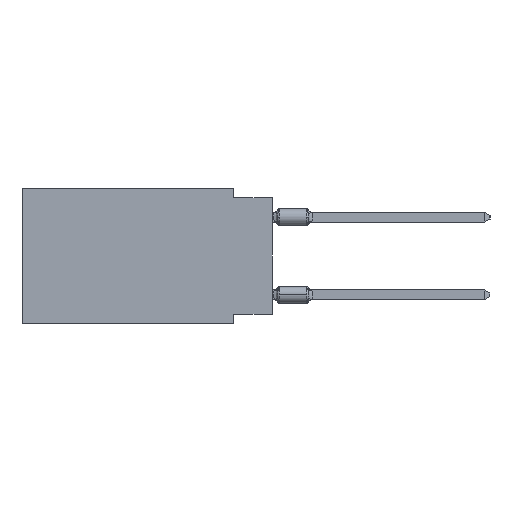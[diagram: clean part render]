
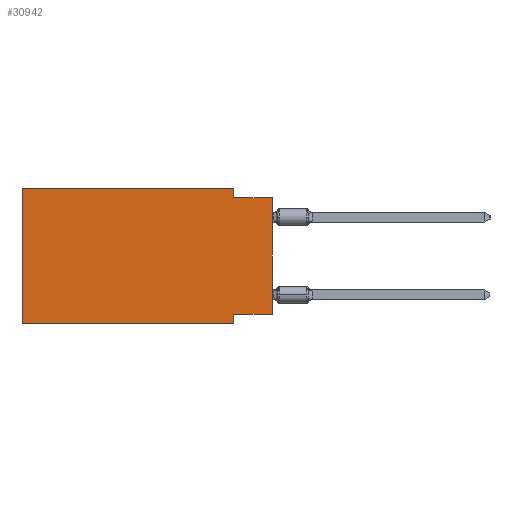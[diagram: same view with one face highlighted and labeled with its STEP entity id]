
A CAD part, left-side view. The second image highlights one B-rep face of the part: STEP entity #30942.
In plain terms, the highlighted planar face has unit normal (-1, 0, 0).
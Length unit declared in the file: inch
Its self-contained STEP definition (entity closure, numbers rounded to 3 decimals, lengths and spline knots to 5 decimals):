
#561 = AXIS2_PLACEMENT_3D ( 'NONE', #1893, #31019, #17840 ) ;
#577 = EDGE_CURVE ( 'NONE', #6546, #15256, #30887, .T. ) ;
#796 = EDGE_CURVE ( 'NONE', #6546, #3663, #32170, .T. ) ;
#1893 = CARTESIAN_POINT ( 'NONE',  ( 0., 0.645, 0. ) ) ;
#2189 = EDGE_LOOP ( 'NONE', ( #30803, #37781, #32144, #37199, #9727, #32442, #23612, #23985 ) ) ;
#2251 = CARTESIAN_POINT ( 'NONE',  ( 0., 0.645, -0.35 ) ) ;
#3054 = EDGE_CURVE ( 'NONE', #3663, #24401, #9322, .T. ) ;
#3663 = VERTEX_POINT ( 'NONE', #26850 ) ;
#4867 = FACE_OUTER_BOUND ( 'NONE', #2189, .T. ) ;
#5063 = DIRECTION ( 'NONE',  ( 0., 0., -1. ) ) ;
#6546 = VERTEX_POINT ( 'NONE', #2251 ) ;
#7403 = VECTOR ( 'NONE', #8085, 39.37008 ) ;
#8085 = DIRECTION ( 'NONE',  ( 0., 1., 0. ) ) ;
#9322 = LINE ( 'NONE', #28452, #16639 ) ;
#9586 = CARTESIAN_POINT ( 'NONE',  ( 0., 0.1, -0.025 ) ) ;
#9727 = ORIENTED_EDGE ( 'NONE', *, *, #796, .F. ) ;
#10822 = DIRECTION ( 'NONE',  ( 0., 0., 1. ) ) ;
#10855 = VECTOR ( 'NONE', #23421, 39.37008 ) ;
#11446 = CARTESIAN_POINT ( 'NONE',  ( 0., 0., 0. ) ) ;
#13526 = DIRECTION ( 'NONE',  ( 0., -1., 0. ) ) ;
#13620 = VERTEX_POINT ( 'NONE', #9586 ) ;
#13847 = CARTESIAN_POINT ( 'NONE',  ( 0., 0.645, 0. ) ) ;
#14323 = VECTOR ( 'NONE', #10822, 39.37008 ) ;
#14880 = VERTEX_POINT ( 'NONE', #41095 ) ;
#15256 = VERTEX_POINT ( 'NONE', #16311 ) ;
#15702 = DIRECTION ( 'NONE',  ( 0., -1., 0. ) ) ;
#16311 = CARTESIAN_POINT ( 'NONE',  ( 0., 0.1, -0.35 ) ) ;
#16639 = VECTOR ( 'NONE', #15702, 39.37008 ) ;
#17840 = DIRECTION ( 'NONE',  ( 0., 0., -1. ) ) ;
#17915 = CARTESIAN_POINT ( 'NONE',  ( 0., 0.645, -0.35 ) ) ;
#19851 = DIRECTION ( 'NONE',  ( 0., 0., -1. ) ) ;
#20159 = EDGE_CURVE ( 'NONE', #40068, #14880, #28040, .T. ) ;
#22267 = CARTESIAN_POINT ( 'NONE',  ( 0., 0.1, 0. ) ) ;
#23302 = VECTOR ( 'NONE', #40716, 39.37008 ) ;
#23421 = DIRECTION ( 'NONE',  ( 0., 0., 1. ) ) ;
#23612 = ORIENTED_EDGE ( 'NONE', *, *, #24931, .F. ) ;
#23822 = VERTEX_POINT ( 'NONE', #23880 ) ;
#23880 = CARTESIAN_POINT ( 'NONE',  ( 0., 0., -0.025 ) ) ;
#23985 = ORIENTED_EDGE ( 'NONE', *, *, #20159, .F. ) ;
#24401 = VERTEX_POINT ( 'NONE', #22267 ) ;
#24602 = EDGE_CURVE ( 'NONE', #13620, #23822, #33918, .T. ) ;
#24644 = CARTESIAN_POINT ( 'NONE',  ( 0., 0.1, 0. ) ) ;
#24931 = EDGE_CURVE ( 'NONE', #14880, #15256, #26621, .T. ) ;
#26621 = LINE ( 'NONE', #33638, #40523 ) ;
#26850 = CARTESIAN_POINT ( 'NONE',  ( 0., 0.645, 0. ) ) ;
#27182 = VECTOR ( 'NONE', #5063, 39.37008 ) ;
#28040 = LINE ( 'NONE', #37884, #7403 ) ;
#28452 = CARTESIAN_POINT ( 'NONE',  ( 0., 0.645, 0. ) ) ;
#30803 = ORIENTED_EDGE ( 'NONE', *, *, #34130, .T. ) ;
#30887 = LINE ( 'NONE', #17915, #23302 ) ;
#30942 = ADVANCED_FACE ( 'NONE', ( #4867 ), #36997, .F. ) ;
#31010 = LINE ( 'NONE', #11446, #14323 ) ;
#31019 = DIRECTION ( 'NONE',  ( 1., 0., 0. ) ) ;
#32144 = ORIENTED_EDGE ( 'NONE', *, *, #35054, .F. ) ;
#32170 = LINE ( 'NONE', #13847, #10855 ) ;
#32442 = ORIENTED_EDGE ( 'NONE', *, *, #577, .T. ) ;
#32872 = CARTESIAN_POINT ( 'NONE',  ( 0., 0., -0.325 ) ) ;
#33296 = CARTESIAN_POINT ( 'NONE',  ( 0., 0., -0.025 ) ) ;
#33638 = CARTESIAN_POINT ( 'NONE',  ( 0., 0.1, -0.35 ) ) ;
#33918 = LINE ( 'NONE', #33296, #36460 ) ;
#34011 = LINE ( 'NONE', #24644, #27182 ) ;
#34130 = EDGE_CURVE ( 'NONE', #40068, #23822, #31010, .T. ) ;
#35054 = EDGE_CURVE ( 'NONE', #24401, #13620, #34011, .T. ) ;
#36460 = VECTOR ( 'NONE', #13526, 39.37008 ) ;
#36997 = PLANE ( 'NONE',  #561 ) ;
#37199 = ORIENTED_EDGE ( 'NONE', *, *, #3054, .F. ) ;
#37781 = ORIENTED_EDGE ( 'NONE', *, *, #24602, .F. ) ;
#37884 = CARTESIAN_POINT ( 'NONE',  ( 0., 0., -0.325 ) ) ;
#40068 = VERTEX_POINT ( 'NONE', #32872 ) ;
#40523 = VECTOR ( 'NONE', #19851, 39.37008 ) ;
#40716 = DIRECTION ( 'NONE',  ( 0., -1., 0. ) ) ;
#41095 = CARTESIAN_POINT ( 'NONE',  ( 0., 0.1, -0.325 ) ) ;
